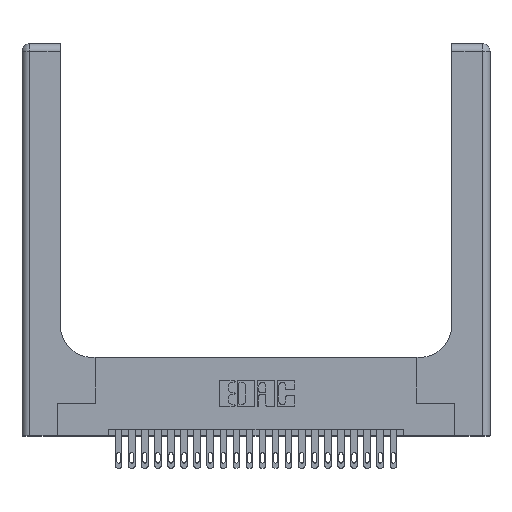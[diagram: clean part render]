
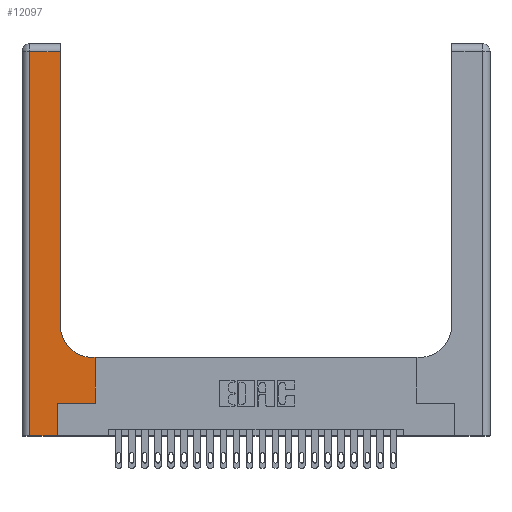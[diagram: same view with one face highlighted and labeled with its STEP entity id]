
A CAD part, top view. The second image highlights one B-rep face of the part: STEP entity #12097.
In plain terms, the highlighted planar face has unit normal (0, 0, 1).
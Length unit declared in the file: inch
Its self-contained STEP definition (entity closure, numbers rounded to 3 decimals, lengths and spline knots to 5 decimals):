
#541 = EDGE_CURVE ( 'NONE', #4643, #6655, #21002, .T. ) ;
#754 = CARTESIAN_POINT ( 'NONE',  ( 0., 3., 0.37 ) ) ;
#1154 = VECTOR ( 'NONE', #24319, 39.37008 ) ;
#1187 = CARTESIAN_POINT ( 'NONE',  ( 0.269, 0., 0.37 ) ) ;
#1573 = DIRECTION ( 'NONE',  ( 1., 0., 0. ) ) ;
#1853 = CARTESIAN_POINT ( 'NONE',  ( 0.5585, 0.25, 0.37 ) ) ;
#2282 = AXIS2_PLACEMENT_3D ( 'NONE', #15557, #2442, #1573 ) ;
#2348 = VERTEX_POINT ( 'NONE', #11205 ) ;
#2442 = DIRECTION ( 'NONE',  ( 0., 0., -1. ) ) ;
#2996 = LINE ( 'NONE', #16469, #1154 ) ;
#3014 = CARTESIAN_POINT ( 'NONE',  ( 0.2915, 3., 0.37 ) ) ;
#3336 = DIRECTION ( 'NONE',  ( 1., 0., 0. ) ) ;
#4070 = VECTOR ( 'NONE', #18564, 39.37008 ) ;
#4527 = VECTOR ( 'NONE', #15798, 39.37008 ) ;
#4528 = DIRECTION ( 'NONE',  ( 0., 1., 0. ) ) ;
#4643 = VERTEX_POINT ( 'NONE', #12422 ) ;
#5125 = LINE ( 'NONE', #12024, #4527 ) ;
#5765 = LINE ( 'NONE', #1853, #20596 ) ;
#6467 = VECTOR ( 'NONE', #12102, 39.37008 ) ;
#6655 = VERTEX_POINT ( 'NONE', #10518 ) ;
#6725 = DIRECTION ( 'NONE',  ( 0., 0., -1. ) ) ;
#7675 = ORIENTED_EDGE ( 'NONE', *, *, #18184, .T. ) ;
#8357 = EDGE_CURVE ( 'NONE', #20412, #16060, #22198, .T. ) ;
#8662 = DIRECTION ( 'NONE',  ( -1., 0., 0. ) ) ;
#8724 = FACE_OUTER_BOUND ( 'NONE', #17776, .T. ) ;
#8744 = ORIENTED_EDGE ( 'NONE', *, *, #19033, .T. ) ;
#9049 = AXIS2_PLACEMENT_3D ( 'NONE', #754, #6725, #8662 ) ;
#9255 = EDGE_CURVE ( 'NONE', #12204, #17489, #23070, .T. ) ;
#9647 = CARTESIAN_POINT ( 'NONE',  ( 0.06, 3., 0.37 ) ) ;
#9756 = CARTESIAN_POINT ( 'NONE',  ( 0.269, 0., 0.37 ) ) ;
#10209 = EDGE_CURVE ( 'NONE', #17489, #2348, #12452, .T. ) ;
#10518 = CARTESIAN_POINT ( 'NONE',  ( 0.06, 0., 0.37 ) ) ;
#10542 = ORIENTED_EDGE ( 'NONE', *, *, #9255, .T. ) ;
#10699 = CARTESIAN_POINT ( 'NONE',  ( 0.2915, 0.6, 0.37 ) ) ;
#10704 = PLANE ( 'NONE',  #9049 ) ;
#11036 = CARTESIAN_POINT ( 'NONE',  ( 0.2915, 0.85, 0.37 ) ) ;
#11205 = CARTESIAN_POINT ( 'NONE',  ( 0.5585, 0.25, 0.37 ) ) ;
#11225 = EDGE_CURVE ( 'NONE', #6655, #12204, #5125, .T. ) ;
#11467 = EDGE_CURVE ( 'NONE', #22694, #14882, #16608, .T. ) ;
#11536 = CARTESIAN_POINT ( 'NONE',  ( 0.269, 0.25, 0.37 ) ) ;
#11864 = CIRCLE ( 'NONE', #2282, 0.25 ) ;
#12020 = ORIENTED_EDGE ( 'NONE', *, *, #8357, .T. ) ;
#12024 = CARTESIAN_POINT ( 'NONE',  ( 0., 0., 0.37 ) ) ;
#12097 = ADVANCED_FACE ( 'NONE', ( #8724 ), #10704, .F. ) ;
#12102 = DIRECTION ( 'NONE',  ( 0., -1., 0. ) ) ;
#12204 = VERTEX_POINT ( 'NONE', #1187 ) ;
#12422 = CARTESIAN_POINT ( 'NONE',  ( 0.06, 2.94, 0.37 ) ) ;
#12452 = LINE ( 'NONE', #24466, #23313 ) ;
#12956 = ORIENTED_EDGE ( 'NONE', *, *, #11225, .T. ) ;
#13301 = VECTOR ( 'NONE', #16725, 39.37008 ) ;
#14882 = VERTEX_POINT ( 'NONE', #24278 ) ;
#15192 = ORIENTED_EDGE ( 'NONE', *, *, #541, .T. ) ;
#15194 = ORIENTED_EDGE ( 'NONE', *, *, #10209, .T. ) ;
#15557 = CARTESIAN_POINT ( 'NONE',  ( 0.5415, 0.85, 0.37 ) ) ;
#15702 = ORIENTED_EDGE ( 'NONE', *, *, #11467, .T. ) ;
#15798 = DIRECTION ( 'NONE',  ( 1., 0., 0. ) ) ;
#15960 = ORIENTED_EDGE ( 'NONE', *, *, #18518, .T. ) ;
#16060 = VERTEX_POINT ( 'NONE', #16905 ) ;
#16469 = CARTESIAN_POINT ( 'NONE',  ( 0., 2.94, 0.37 ) ) ;
#16608 = LINE ( 'NONE', #3014, #13301 ) ;
#16664 = CARTESIAN_POINT ( 'NONE',  ( 0.5585, 0.6, 0.37 ) ) ;
#16725 = DIRECTION ( 'NONE',  ( 0., 1., 0. ) ) ;
#16905 = CARTESIAN_POINT ( 'NONE',  ( 0.5415, 0.6, 0.37 ) ) ;
#17489 = VERTEX_POINT ( 'NONE', #11536 ) ;
#17776 = EDGE_LOOP ( 'NONE', ( #15702, #8744, #15192, #12956, #10542, #15194, #15960, #12020, #7675 ) ) ;
#17957 = VECTOR ( 'NONE', #4528, 39.37008 ) ;
#18184 = EDGE_CURVE ( 'NONE', #16060, #22694, #11864, .T. ) ;
#18518 = EDGE_CURVE ( 'NONE', #2348, #20412, #5765, .T. ) ;
#18564 = DIRECTION ( 'NONE',  ( -1., 0., 0. ) ) ;
#19033 = EDGE_CURVE ( 'NONE', #14882, #4643, #2996, .T. ) ;
#20412 = VERTEX_POINT ( 'NONE', #16664 ) ;
#20596 = VECTOR ( 'NONE', #24923, 39.37008 ) ;
#21002 = LINE ( 'NONE', #9647, #6467 ) ;
#22198 = LINE ( 'NONE', #10699, #4070 ) ;
#22694 = VERTEX_POINT ( 'NONE', #11036 ) ;
#23070 = LINE ( 'NONE', #9756, #17957 ) ;
#23313 = VECTOR ( 'NONE', #3336, 39.37008 ) ;
#24278 = CARTESIAN_POINT ( 'NONE',  ( 0.2915, 2.94, 0.37 ) ) ;
#24319 = DIRECTION ( 'NONE',  ( -1., 0., 0. ) ) ;
#24466 = CARTESIAN_POINT ( 'NONE',  ( 0.269, 0.25, 0.37 ) ) ;
#24923 = DIRECTION ( 'NONE',  ( 0., 1., 0. ) ) ;
